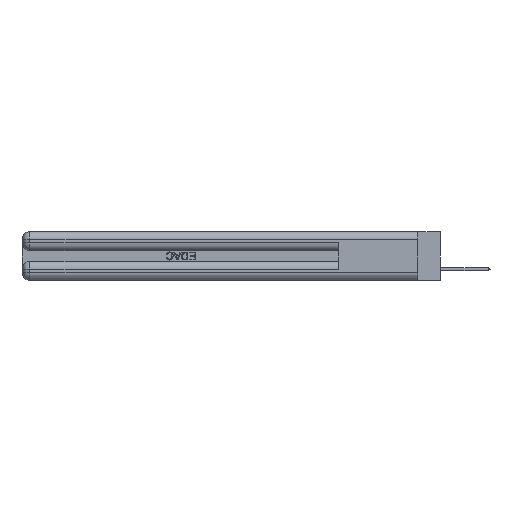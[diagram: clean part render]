
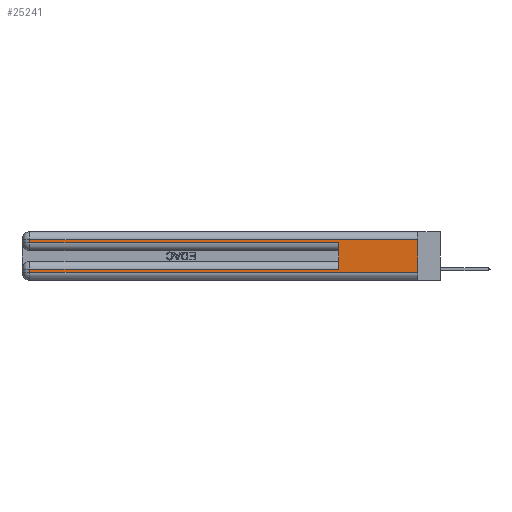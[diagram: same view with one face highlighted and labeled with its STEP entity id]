
A CAD part, left-side view. The second image highlights one B-rep face of the part: STEP entity #25241.
In plain terms, the highlighted planar face has unit normal (-1, 0, 0).
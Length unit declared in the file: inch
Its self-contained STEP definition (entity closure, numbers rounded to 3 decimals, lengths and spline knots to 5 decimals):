
#246 = EDGE_CURVE ( 'NONE', #8901, #20894, #41170, .T. ) ;
#1223 = EDGE_CURVE ( 'NONE', #8320, #7814, #25800, .T. ) ;
#2626 = PLANE ( 'NONE',  #37769 ) ;
#3821 = VECTOR ( 'NONE', #40653, 39.37008 ) ;
#3822 = VECTOR ( 'NONE', #48148, 39.37008 ) ;
#5845 = DIRECTION ( 'NONE',  ( 0., -1., 0. ) ) ;
#6589 = DIRECTION ( 'NONE',  ( 1., 0., 0. ) ) ;
#7312 = CARTESIAN_POINT ( 'NONE',  ( 0., 2.94, 0.37 ) ) ;
#7328 = ORIENTED_EDGE ( 'NONE', *, *, #10000, .F. ) ;
#7814 = VERTEX_POINT ( 'NONE', #45267 ) ;
#7973 = ORIENTED_EDGE ( 'NONE', *, *, #246, .T. ) ;
#8061 = ORIENTED_EDGE ( 'NONE', *, *, #26782, .T. ) ;
#8177 = LINE ( 'NONE', #25288, #36239 ) ;
#8218 = EDGE_CURVE ( 'NONE', #20894, #10449, #8177, .T. ) ;
#8320 = VERTEX_POINT ( 'NONE', #49343 ) ;
#8901 = VERTEX_POINT ( 'NONE', #10200 ) ;
#10000 = EDGE_CURVE ( 'NONE', #30152, #10449, #50069, .T. ) ;
#10200 = CARTESIAN_POINT ( 'NONE',  ( 0., 2.94, 0.31 ) ) ;
#10349 = LINE ( 'NONE', #11525, #23213 ) ;
#10449 = VERTEX_POINT ( 'NONE', #49260 ) ;
#10637 = CARTESIAN_POINT ( 'NONE',  ( 0., 2.94, 0.37 ) ) ;
#11525 = CARTESIAN_POINT ( 'NONE',  ( 0., 0., 0.06 ) ) ;
#14591 = DIRECTION ( 'NONE',  ( 0., 0., -1. ) ) ;
#15207 = VECTOR ( 'NONE', #27341, 39.37008 ) ;
#17542 = LINE ( 'NONE', #7312, #18808 ) ;
#18808 = VECTOR ( 'NONE', #43586, 39.37008 ) ;
#18969 = VECTOR ( 'NONE', #30045, 39.37008 ) ;
#20894 = VERTEX_POINT ( 'NONE', #37623 ) ;
#21892 = CARTESIAN_POINT ( 'NONE',  ( 0., 0., 0.085 ) ) ;
#23165 = VERTEX_POINT ( 'NONE', #44104 ) ;
#23213 = VECTOR ( 'NONE', #30521, 39.37008 ) ;
#24547 = ORIENTED_EDGE ( 'NONE', *, *, #36616, .T. ) ;
#25241 = ADVANCED_FACE ( 'NONE', ( #31158 ), #2626, .F. ) ;
#25288 = CARTESIAN_POINT ( 'NONE',  ( 0., 0., 0.285 ) ) ;
#25800 = LINE ( 'NONE', #28610, #3822 ) ;
#26014 = CARTESIAN_POINT ( 'NONE',  ( 0., 0.6, 0.085 ) ) ;
#26512 = VERTEX_POINT ( 'NONE', #49395 ) ;
#26572 = DIRECTION ( 'NONE',  ( 0., 0., -1. ) ) ;
#26782 = EDGE_CURVE ( 'NONE', #30152, #23165, #35002, .T. ) ;
#27341 = DIRECTION ( 'NONE',  ( 0., 1., 0. ) ) ;
#28610 = CARTESIAN_POINT ( 'NONE',  ( 0., 0., 0.37 ) ) ;
#29234 = EDGE_CURVE ( 'NONE', #23165, #26512, #17542, .T. ) ;
#29664 = CARTESIAN_POINT ( 'NONE',  ( 0., 0., 0.37 ) ) ;
#30045 = DIRECTION ( 'NONE',  ( 0., 0., 1. ) ) ;
#30152 = VERTEX_POINT ( 'NONE', #26014 ) ;
#30521 = DIRECTION ( 'NONE',  ( 0., -1., 0. ) ) ;
#31028 = ORIENTED_EDGE ( 'NONE', *, *, #8218, .T. ) ;
#31158 = FACE_OUTER_BOUND ( 'NONE', #43180, .T. ) ;
#31428 = VECTOR ( 'NONE', #14591, 39.37008 ) ;
#32297 = ORIENTED_EDGE ( 'NONE', *, *, #45458, .T. ) ;
#35002 = LINE ( 'NONE', #21892, #3821 ) ;
#36239 = VECTOR ( 'NONE', #5845, 39.37008 ) ;
#36616 = EDGE_CURVE ( 'NONE', #8320, #8901, #49105, .T. ) ;
#37623 = CARTESIAN_POINT ( 'NONE',  ( 0., 2.94, 0.285 ) ) ;
#37769 = AXIS2_PLACEMENT_3D ( 'NONE', #29664, #6589, #26572 ) ;
#39331 = CARTESIAN_POINT ( 'NONE',  ( 0., 0.6, 0.145 ) ) ;
#40653 = DIRECTION ( 'NONE',  ( 0., 1., 0. ) ) ;
#41170 = LINE ( 'NONE', #10637, #31428 ) ;
#43180 = EDGE_LOOP ( 'NONE', ( #47322, #24547, #7973, #31028, #7328, #8061, #45966, #32297 ) ) ;
#43586 = DIRECTION ( 'NONE',  ( 0., 0., -1. ) ) ;
#44104 = CARTESIAN_POINT ( 'NONE',  ( 0., 2.94, 0.085 ) ) ;
#45267 = CARTESIAN_POINT ( 'NONE',  ( 0., 0., 0.06 ) ) ;
#45458 = EDGE_CURVE ( 'NONE', #26512, #7814, #10349, .T. ) ;
#45966 = ORIENTED_EDGE ( 'NONE', *, *, #29234, .T. ) ;
#47322 = ORIENTED_EDGE ( 'NONE', *, *, #1223, .F. ) ;
#48148 = DIRECTION ( 'NONE',  ( 0., 0., -1. ) ) ;
#49105 = LINE ( 'NONE', #50481, #15207 ) ;
#49260 = CARTESIAN_POINT ( 'NONE',  ( 0., 0.6, 0.285 ) ) ;
#49343 = CARTESIAN_POINT ( 'NONE',  ( 0., 0., 0.31 ) ) ;
#49395 = CARTESIAN_POINT ( 'NONE',  ( 0., 2.94, 0.06 ) ) ;
#50069 = LINE ( 'NONE', #39331, #18969 ) ;
#50481 = CARTESIAN_POINT ( 'NONE',  ( 0., 0., 0.31 ) ) ;
